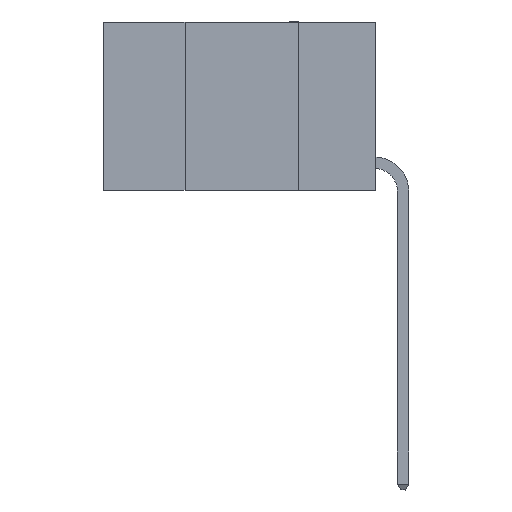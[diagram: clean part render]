
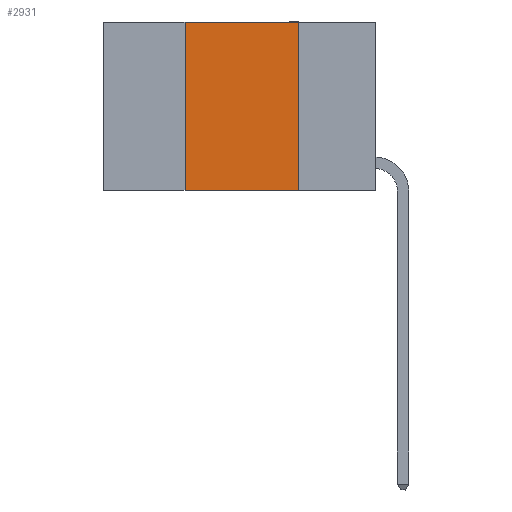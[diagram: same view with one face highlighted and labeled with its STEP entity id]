
A CAD part, left-side view. The second image highlights one B-rep face of the part: STEP entity #2931.
In plain terms, the highlighted planar face has unit normal (-1, 0, 0).
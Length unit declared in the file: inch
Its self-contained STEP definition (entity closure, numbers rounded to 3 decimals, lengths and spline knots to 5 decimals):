
#321 = VERTEX_POINT ( 'NONE', #9968 ) ;
#1187 = ORIENTED_EDGE ( 'NONE', *, *, #21586, .F. ) ;
#1741 = ORIENTED_EDGE ( 'NONE', *, *, #16460, .F. ) ;
#2931 = ADVANCED_FACE ( 'NONE', ( #20746 ), #14374, .F. ) ;
#4225 = VERTEX_POINT ( 'NONE', #19652 ) ;
#4251 = CARTESIAN_POINT ( 'NONE',  ( 0., 0.6, 0. ) ) ;
#4579 = VECTOR ( 'NONE', #18849, 39.37008 ) ;
#4744 = LINE ( 'NONE', #9445, #21484 ) ;
#7220 = CARTESIAN_POINT ( 'NONE',  ( 0., 0.17, 0. ) ) ;
#7592 = CARTESIAN_POINT ( 'NONE',  ( 0., 0.42, 0. ) ) ;
#7752 = DIRECTION ( 'NONE',  ( 0., -1., 0. ) ) ;
#7758 = DIRECTION ( 'NONE',  ( 0., 0., -1. ) ) ;
#8838 = CARTESIAN_POINT ( 'NONE',  ( 0., 0.6, -0.37 ) ) ;
#9274 = ORIENTED_EDGE ( 'NONE', *, *, #13623, .T. ) ;
#9284 = DIRECTION ( 'NONE',  ( 0., 0., 1. ) ) ;
#9445 = CARTESIAN_POINT ( 'NONE',  ( 0., 0.6, 0. ) ) ;
#9968 = CARTESIAN_POINT ( 'NONE',  ( 0., 0.42, -0.37 ) ) ;
#11130 = LINE ( 'NONE', #15069, #15037 ) ;
#13493 = LINE ( 'NONE', #8838, #4579 ) ;
#13594 = VECTOR ( 'NONE', #9284, 39.37008 ) ;
#13623 = EDGE_CURVE ( 'NONE', #321, #21686, #13493, .T. ) ;
#14228 = EDGE_LOOP ( 'NONE', ( #1187, #1741, #18170, #9274 ) ) ;
#14374 = PLANE ( 'NONE',  #21473 ) ;
#15037 = VECTOR ( 'NONE', #16760, 39.37008 ) ;
#15069 = CARTESIAN_POINT ( 'NONE',  ( 0., 0.17, 0. ) ) ;
#16460 = EDGE_CURVE ( 'NONE', #4225, #17697, #4744, .T. ) ;
#16760 = DIRECTION ( 'NONE',  ( 0., 0., -1. ) ) ;
#16987 = CARTESIAN_POINT ( 'NONE',  ( 0., 0.17, -0.37 ) ) ;
#17697 = VERTEX_POINT ( 'NONE', #7220 ) ;
#17771 = DIRECTION ( 'NONE',  ( 1., 0., 0. ) ) ;
#17850 = EDGE_CURVE ( 'NONE', #321, #4225, #18623, .T. ) ;
#18170 = ORIENTED_EDGE ( 'NONE', *, *, #17850, .F. ) ;
#18623 = LINE ( 'NONE', #7592, #13594 ) ;
#18849 = DIRECTION ( 'NONE',  ( 0., -1., 0. ) ) ;
#19652 = CARTESIAN_POINT ( 'NONE',  ( 0., 0.42, 0. ) ) ;
#20746 = FACE_OUTER_BOUND ( 'NONE', #14228, .T. ) ;
#21473 = AXIS2_PLACEMENT_3D ( 'NONE', #4251, #17771, #7758 ) ;
#21484 = VECTOR ( 'NONE', #7752, 39.37008 ) ;
#21586 = EDGE_CURVE ( 'NONE', #17697, #21686, #11130, .T. ) ;
#21686 = VERTEX_POINT ( 'NONE', #16987 ) ;
